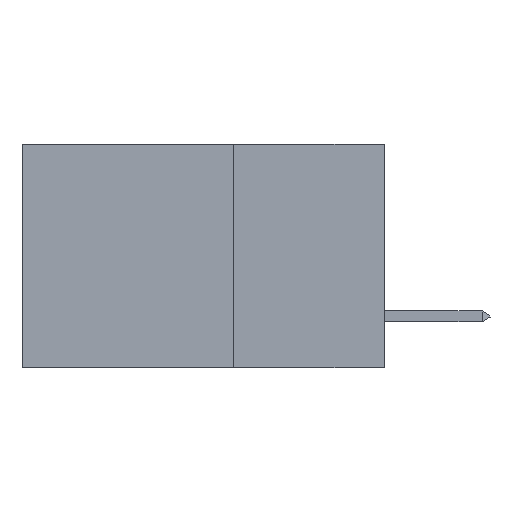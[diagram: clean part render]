
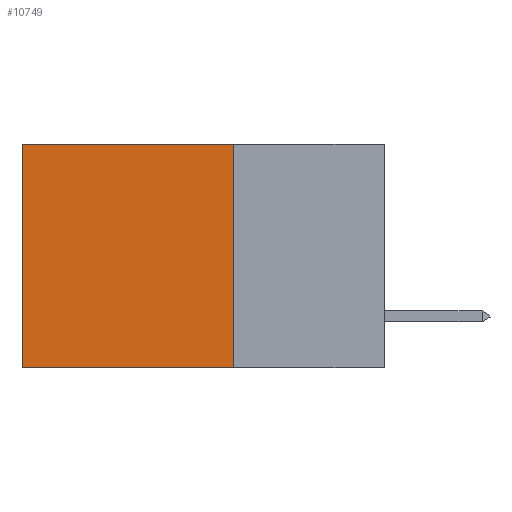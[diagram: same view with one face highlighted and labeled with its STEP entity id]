
A CAD part, left-side view. The second image highlights one B-rep face of the part: STEP entity #10749.
In plain terms, the highlighted planar face has unit normal (-1, 0, 0).
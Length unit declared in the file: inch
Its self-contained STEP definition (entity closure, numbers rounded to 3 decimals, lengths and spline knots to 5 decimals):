
#502 = LINE ( 'NONE', #11471, #15418 ) ;
#1294 = AXIS2_PLACEMENT_3D ( 'NONE', #8455, #2564, #4967 ) ;
#2199 = VECTOR ( 'NONE', #10706, 39.37008 ) ;
#2452 = EDGE_CURVE ( 'NONE', #6215, #7342, #5414, .T. ) ;
#2564 = DIRECTION ( 'NONE',  ( 1., 0., 0. ) ) ;
#2680 = VECTOR ( 'NONE', #10560, 39.37008 ) ;
#3149 = CARTESIAN_POINT ( 'NONE',  ( 0.2875, 0.6, 0. ) ) ;
#4816 = CARTESIAN_POINT ( 'NONE',  ( 0.2875, 0.25, 0. ) ) ;
#4967 = DIRECTION ( 'NONE',  ( 0., 0., -1. ) ) ;
#5036 = CARTESIAN_POINT ( 'NONE',  ( 0.2875, 0.25, 0. ) ) ;
#5414 = LINE ( 'NONE', #4816, #2199 ) ;
#5797 = FACE_OUTER_BOUND ( 'NONE', #14425, .T. ) ;
#6215 = VERTEX_POINT ( 'NONE', #13814 ) ;
#6403 = DIRECTION ( 'NONE',  ( 0., 0., -1. ) ) ;
#6861 = LINE ( 'NONE', #15072, #2680 ) ;
#7203 = VERTEX_POINT ( 'NONE', #10279 ) ;
#7234 = PLANE ( 'NONE',  #1294 ) ;
#7342 = VERTEX_POINT ( 'NONE', #3149 ) ;
#8455 = CARTESIAN_POINT ( 'NONE',  ( 0.2875, 0.25, 0. ) ) ;
#8717 = VERTEX_POINT ( 'NONE', #10076 ) ;
#8987 = DIRECTION ( 'NONE',  ( 0., 1., 0. ) ) ;
#9145 = ORIENTED_EDGE ( 'NONE', *, *, #13962, .T. ) ;
#10076 = CARTESIAN_POINT ( 'NONE',  ( 0.2875, 0.25, -0.37 ) ) ;
#10264 = ORIENTED_EDGE ( 'NONE', *, *, #2452, .T. ) ;
#10279 = CARTESIAN_POINT ( 'NONE',  ( 0.2875, 0.6, -0.37 ) ) ;
#10560 = DIRECTION ( 'NONE',  ( 0., 0., -1. ) ) ;
#10706 = DIRECTION ( 'NONE',  ( 0., 1., 0. ) ) ;
#10749 = ADVANCED_FACE ( 'NONE', ( #5797 ), #7234, .F. ) ;
#10958 = ORIENTED_EDGE ( 'NONE', *, *, #15597, .F. ) ;
#10988 = EDGE_CURVE ( 'NONE', #8717, #7203, #502, .T. ) ;
#11360 = LINE ( 'NONE', #5036, #15315 ) ;
#11471 = CARTESIAN_POINT ( 'NONE',  ( 0.2875, 0.25, -0.37 ) ) ;
#12770 = ORIENTED_EDGE ( 'NONE', *, *, #10988, .F. ) ;
#13814 = CARTESIAN_POINT ( 'NONE',  ( 0.2875, 0.25, 0. ) ) ;
#13962 = EDGE_CURVE ( 'NONE', #7342, #7203, #6861, .T. ) ;
#14425 = EDGE_LOOP ( 'NONE', ( #9145, #12770, #10958, #10264 ) ) ;
#15072 = CARTESIAN_POINT ( 'NONE',  ( 0.2875, 0.6, 0. ) ) ;
#15315 = VECTOR ( 'NONE', #6403, 39.37008 ) ;
#15418 = VECTOR ( 'NONE', #8987, 39.37008 ) ;
#15597 = EDGE_CURVE ( 'NONE', #6215, #8717, #11360, .T. ) ;
